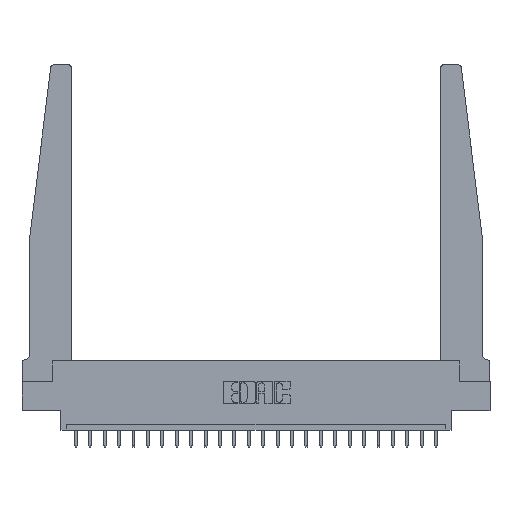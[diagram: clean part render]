
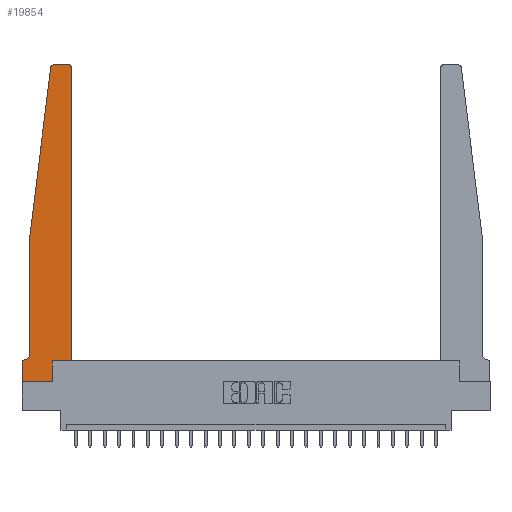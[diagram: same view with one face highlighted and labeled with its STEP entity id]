
A CAD part, top view. The second image highlights one B-rep face of the part: STEP entity #19854.
In plain terms, the highlighted planar face has unit normal (0, 0, 1).
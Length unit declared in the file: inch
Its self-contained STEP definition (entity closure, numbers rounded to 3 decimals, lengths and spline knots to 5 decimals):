
#181 = DIRECTION ( 'NONE',  ( -1., 0., 0. ) ) ;
#373 = LINE ( 'NONE', #4291, #18048 ) ;
#566 = LINE ( 'NONE', #18835, #3789 ) ;
#884 = CARTESIAN_POINT ( 'NONE',  ( 0.2605, 0., 0.37 ) ) ;
#920 = CARTESIAN_POINT ( 'NONE',  ( 0.065, 1.25, 0.37 ) ) ;
#969 = EDGE_CURVE ( 'NONE', #17052, #3218, #5327, .T. ) ;
#1590 = CARTESIAN_POINT ( 'NONE',  ( 0.395, 2.72, 0.37 ) ) ;
#1634 = CARTESIAN_POINT ( 'NONE',  ( 0.065, 0.2375, 0.37 ) ) ;
#1658 = ORIENTED_EDGE ( 'NONE', *, *, #21691, .T. ) ;
#1819 = DIRECTION ( 'NONE',  ( 0., 0., 1. ) ) ;
#1850 = CARTESIAN_POINT ( 'NONE',  ( 0.015, 0.2375, 0.37 ) ) ;
#2231 = LINE ( 'NONE', #11076, #10017 ) ;
#3119 = CARTESIAN_POINT ( 'NONE',  ( 0., 0.1875, 0.37 ) ) ;
#3218 = VERTEX_POINT ( 'NONE', #3119 ) ;
#3741 = VERTEX_POINT ( 'NONE', #15742 ) ;
#3745 = AXIS2_PLACEMENT_3D ( 'NONE', #1850, #7568, #181 ) ;
#3789 = VECTOR ( 'NONE', #7855, 39.37008 ) ;
#4064 = LINE ( 'NONE', #11357, #22383 ) ;
#4291 = CARTESIAN_POINT ( 'NONE',  ( 0.065, 1.25, 0.37 ) ) ;
#4400 = LINE ( 'NONE', #15377, #10330 ) ;
#4523 = ORIENTED_EDGE ( 'NONE', *, *, #15087, .T. ) ;
#4724 = EDGE_CURVE ( 'NONE', #9112, #17052, #7197, .T. ) ;
#4886 = VERTEX_POINT ( 'NONE', #884 ) ;
#5140 = PLANE ( 'NONE',  #10974 ) ;
#5240 = ORIENTED_EDGE ( 'NONE', *, *, #12992, .T. ) ;
#5327 = LINE ( 'NONE', #11056, #14547 ) ;
#5536 = ORIENTED_EDGE ( 'NONE', *, *, #4724, .T. ) ;
#5635 = LINE ( 'NONE', #20211, #15874 ) ;
#5677 = CARTESIAN_POINT ( 'NONE',  ( 0.425, 0.18, 0.37 ) ) ;
#7197 = CIRCLE ( 'NONE', #3745, 0.05 ) ;
#7380 = DIRECTION ( 'NONE',  ( 1., 0., 0. ) ) ;
#7568 = DIRECTION ( 'NONE',  ( 0., 0., -1. ) ) ;
#7770 = ORIENTED_EDGE ( 'NONE', *, *, #9624, .T. ) ;
#7855 = DIRECTION ( 'NONE',  ( 0., -1., 0. ) ) ;
#8102 = ORIENTED_EDGE ( 'NONE', *, *, #16506, .T. ) ;
#8421 = ORIENTED_EDGE ( 'NONE', *, *, #11866, .T. ) ;
#8867 = CARTESIAN_POINT ( 'NONE',  ( 0., 0.1875, 0.37 ) ) ;
#9112 = VERTEX_POINT ( 'NONE', #1634 ) ;
#9370 = VERTEX_POINT ( 'NONE', #23020 ) ;
#9531 = ORIENTED_EDGE ( 'NONE', *, *, #17995, .T. ) ;
#9624 = EDGE_CURVE ( 'NONE', #4886, #16887, #4400, .T. ) ;
#9686 = ORIENTED_EDGE ( 'NONE', *, *, #969, .T. ) ;
#10017 = VECTOR ( 'NONE', #7380, 39.37008 ) ;
#10330 = VECTOR ( 'NONE', #11449, 39.37008 ) ;
#10733 = ORIENTED_EDGE ( 'NONE', *, *, #13236, .T. ) ;
#10974 = AXIS2_PLACEMENT_3D ( 'NONE', #8867, #21764, #18159 ) ;
#11056 = CARTESIAN_POINT ( 'NONE',  ( 0.065, 0.1875, 0.37 ) ) ;
#11076 = CARTESIAN_POINT ( 'NONE',  ( 0.425, 0.18, 0.37 ) ) ;
#11175 = EDGE_CURVE ( 'NONE', #19349, #9112, #21578, .T. ) ;
#11357 = CARTESIAN_POINT ( 'NONE',  ( 0., 0., 0.37 ) ) ;
#11449 = DIRECTION ( 'NONE',  ( 0., 1., 0. ) ) ;
#11866 = EDGE_CURVE ( 'NONE', #3741, #19349, #373, .T. ) ;
#12070 = DIRECTION ( 'NONE',  ( -0.122, -0.992, 0. ) ) ;
#12621 = DIRECTION ( 'NONE',  ( -1., 0., 0. ) ) ;
#12713 = DIRECTION ( 'NONE',  ( 0., -1., 0. ) ) ;
#12992 = EDGE_CURVE ( 'NONE', #13962, #16410, #21357, .T. ) ;
#13236 = EDGE_CURVE ( 'NONE', #16410, #19138, #5635, .T. ) ;
#13962 = VERTEX_POINT ( 'NONE', #18479 ) ;
#14122 = ORIENTED_EDGE ( 'NONE', *, *, #11175, .T. ) ;
#14392 = ORIENTED_EDGE ( 'NONE', *, *, #21638, .T. ) ;
#14547 = VECTOR ( 'NONE', #12621, 39.37008 ) ;
#14680 = VECTOR ( 'NONE', #18006, 39.37008 ) ;
#15087 = EDGE_CURVE ( 'NONE', #22070, #13962, #23293, .T. ) ;
#15377 = CARTESIAN_POINT ( 'NONE',  ( 0.2605, 0.18, 0.37 ) ) ;
#15742 = CARTESIAN_POINT ( 'NONE',  ( 0.24675, 2.72367, 0.37 ) ) ;
#15874 = VECTOR ( 'NONE', #16941, 39.37008 ) ;
#15875 = CIRCLE ( 'NONE', #16245, 0.03 ) ;
#16221 = FACE_OUTER_BOUND ( 'NONE', #18499, .T. ) ;
#16245 = AXIS2_PLACEMENT_3D ( 'NONE', #22280, #20473, #20360 ) ;
#16379 = CARTESIAN_POINT ( 'NONE',  ( 0.065, 1.25, 0.37 ) ) ;
#16410 = VERTEX_POINT ( 'NONE', #16513 ) ;
#16506 = EDGE_CURVE ( 'NONE', #19138, #3741, #15875, .T. ) ;
#16513 = CARTESIAN_POINT ( 'NONE',  ( 0.395, 2.75, 0.37 ) ) ;
#16887 = VERTEX_POINT ( 'NONE', #21013 ) ;
#16941 = DIRECTION ( 'NONE',  ( -1., 0., 0. ) ) ;
#17052 = VERTEX_POINT ( 'NONE', #17407 ) ;
#17407 = CARTESIAN_POINT ( 'NONE',  ( 0.015, 0.1875, 0.37 ) ) ;
#17681 = VECTOR ( 'NONE', #12713, 39.37008 ) ;
#17995 = EDGE_CURVE ( 'NONE', #9370, #4886, #4064, .T. ) ;
#18006 = DIRECTION ( 'NONE',  ( 0., 1., 0. ) ) ;
#18048 = VECTOR ( 'NONE', #12070, 39.37008 ) ;
#18118 = CARTESIAN_POINT ( 'NONE',  ( 0.425, 0.18, 0.37 ) ) ;
#18159 = DIRECTION ( 'NONE',  ( 1., 0., 0. ) ) ;
#18479 = CARTESIAN_POINT ( 'NONE',  ( 0.425, 2.72, 0.37 ) ) ;
#18499 = EDGE_LOOP ( 'NONE', ( #10733, #8102, #8421, #14122, #5536, #9686, #1658, #9531, #7770, #14392, #4523, #5240 ) ) ;
#18653 = DIRECTION ( 'NONE',  ( 1., 0., 0. ) ) ;
#18835 = CARTESIAN_POINT ( 'NONE',  ( 0., 0., 0.37 ) ) ;
#19138 = VERTEX_POINT ( 'NONE', #21382 ) ;
#19349 = VERTEX_POINT ( 'NONE', #920 ) ;
#19854 = ADVANCED_FACE ( 'NONE', ( #16221 ), #5140, .T. ) ;
#19987 = DIRECTION ( 'NONE',  ( 1., 0., 0. ) ) ;
#20198 = AXIS2_PLACEMENT_3D ( 'NONE', #1590, #1819, #19987 ) ;
#20211 = CARTESIAN_POINT ( 'NONE',  ( 0.25, 2.75, 0.37 ) ) ;
#20360 = DIRECTION ( 'NONE',  ( 1., 0., 0. ) ) ;
#20473 = DIRECTION ( 'NONE',  ( 0., 0., 1. ) ) ;
#21013 = CARTESIAN_POINT ( 'NONE',  ( 0.2605, 0.18, 0.37 ) ) ;
#21357 = CIRCLE ( 'NONE', #20198, 0.03 ) ;
#21382 = CARTESIAN_POINT ( 'NONE',  ( 0.27653, 2.75, 0.37 ) ) ;
#21578 = LINE ( 'NONE', #16379, #17681 ) ;
#21638 = EDGE_CURVE ( 'NONE', #16887, #22070, #2231, .T. ) ;
#21691 = EDGE_CURVE ( 'NONE', #3218, #9370, #566, .T. ) ;
#21764 = DIRECTION ( 'NONE',  ( 0., 0., 1. ) ) ;
#22070 = VERTEX_POINT ( 'NONE', #5677 ) ;
#22280 = CARTESIAN_POINT ( 'NONE',  ( 0.27653, 2.72, 0.37 ) ) ;
#22383 = VECTOR ( 'NONE', #18653, 39.37008 ) ;
#23020 = CARTESIAN_POINT ( 'NONE',  ( 0., 0., 0.37 ) ) ;
#23293 = LINE ( 'NONE', #18118, #14680 ) ;
